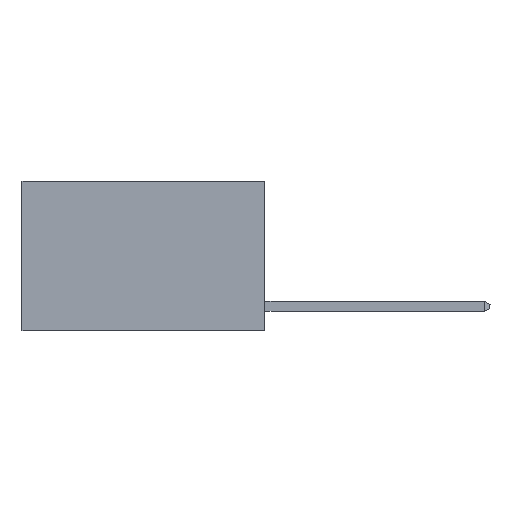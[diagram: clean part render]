
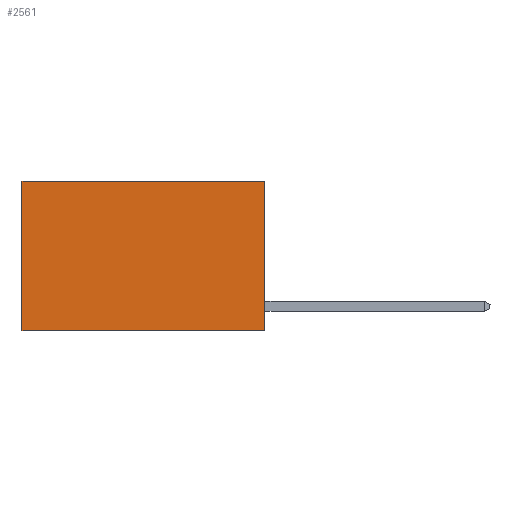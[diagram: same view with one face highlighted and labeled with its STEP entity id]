
A CAD part, left-side view. The second image highlights one B-rep face of the part: STEP entity #2561.
In plain terms, the highlighted planar face has unit normal (-1, 0, 0).
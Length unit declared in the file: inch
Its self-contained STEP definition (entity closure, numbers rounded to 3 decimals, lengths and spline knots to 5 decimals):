
#18 = DIRECTION ( 'NONE',  ( 0., 0., -1. ) ) ;
#1141 = CARTESIAN_POINT ( 'NONE',  ( 0.2625, 0.6, 0. ) ) ;
#1289 = EDGE_CURVE ( 'NONE', #6641, #8532, #7031, .T. ) ;
#1339 = VERTEX_POINT ( 'NONE', #1141 ) ;
#1713 = AXIS2_PLACEMENT_3D ( 'NONE', #5649, #7079, #18 ) ;
#1804 = ORIENTED_EDGE ( 'NONE', *, *, #7727, .T. ) ;
#1968 = EDGE_CURVE ( 'NONE', #8532, #8001, #4207, .T. ) ;
#1999 = DIRECTION ( 'NONE',  ( 0., 1., 0. ) ) ;
#2044 = DIRECTION ( 'NONE',  ( 0., 0., -1. ) ) ;
#2088 = PLANE ( 'NONE',  #1713 ) ;
#2523 = CARTESIAN_POINT ( 'NONE',  ( 0.2625, 0., 0. ) ) ;
#2561 = ADVANCED_FACE ( 'NONE', ( #4881 ), #2088, .F. ) ;
#2564 = CARTESIAN_POINT ( 'NONE',  ( 0.2625, 0.6, -0.37 ) ) ;
#3148 = EDGE_CURVE ( 'NONE', #1339, #8001, #6872, .T. ) ;
#3153 = CARTESIAN_POINT ( 'NONE',  ( 0.2625, 0., 0. ) ) ;
#3247 = EDGE_LOOP ( 'NONE', ( #3320, #4979, #8322, #1804 ) ) ;
#3320 = ORIENTED_EDGE ( 'NONE', *, *, #3148, .T. ) ;
#3979 = VECTOR ( 'NONE', #6749, 39.37008 ) ;
#4207 = LINE ( 'NONE', #7595, #6252 ) ;
#4705 = CARTESIAN_POINT ( 'NONE',  ( 0.2625, 0.6, 0. ) ) ;
#4881 = FACE_OUTER_BOUND ( 'NONE', #3247, .T. ) ;
#4958 = LINE ( 'NONE', #3153, #3979 ) ;
#4979 = ORIENTED_EDGE ( 'NONE', *, *, #1968, .F. ) ;
#5649 = CARTESIAN_POINT ( 'NONE',  ( 0.2625, 0., 0. ) ) ;
#6252 = VECTOR ( 'NONE', #1999, 39.37008 ) ;
#6641 = VERTEX_POINT ( 'NONE', #7345 ) ;
#6749 = DIRECTION ( 'NONE',  ( 0., 1., 0. ) ) ;
#6872 = LINE ( 'NONE', #4705, #8895 ) ;
#7031 = LINE ( 'NONE', #2523, #7369 ) ;
#7079 = DIRECTION ( 'NONE',  ( 1., 0., 0. ) ) ;
#7345 = CARTESIAN_POINT ( 'NONE',  ( 0.2625, 0., 0. ) ) ;
#7369 = VECTOR ( 'NONE', #9043, 39.37008 ) ;
#7595 = CARTESIAN_POINT ( 'NONE',  ( 0.2625, 0., -0.37 ) ) ;
#7727 = EDGE_CURVE ( 'NONE', #6641, #1339, #4958, .T. ) ;
#8001 = VERTEX_POINT ( 'NONE', #2564 ) ;
#8242 = CARTESIAN_POINT ( 'NONE',  ( 0.2625, 0., -0.37 ) ) ;
#8322 = ORIENTED_EDGE ( 'NONE', *, *, #1289, .F. ) ;
#8532 = VERTEX_POINT ( 'NONE', #8242 ) ;
#8895 = VECTOR ( 'NONE', #2044, 39.37008 ) ;
#9043 = DIRECTION ( 'NONE',  ( 0., 0., -1. ) ) ;
